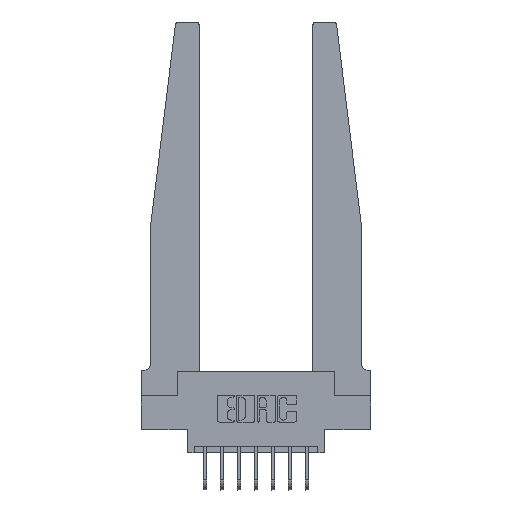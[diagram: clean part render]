
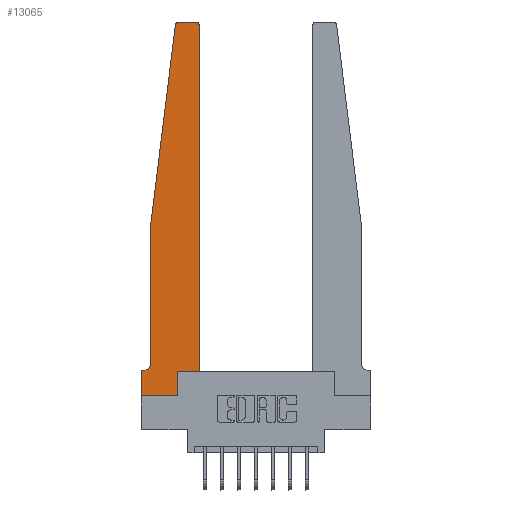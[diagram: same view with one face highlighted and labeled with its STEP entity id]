
A CAD part, top view. The second image highlights one B-rep face of the part: STEP entity #13065.
In plain terms, the highlighted planar face has unit normal (0, 0, 1).
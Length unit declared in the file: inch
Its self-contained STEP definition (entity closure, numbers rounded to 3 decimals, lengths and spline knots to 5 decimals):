
#137 = CARTESIAN_POINT ( 'NONE',  ( 0.425, 0.18, 0.37 ) ) ;
#297 = VERTEX_POINT ( 'NONE', #11031 ) ;
#320 = CIRCLE ( 'NONE', #13896, 0.05 ) ;
#441 = CIRCLE ( 'NONE', #13308, 0.03 ) ;
#601 = CARTESIAN_POINT ( 'NONE',  ( 0.2605, 0., 0.37 ) ) ;
#698 = EDGE_CURVE ( 'NONE', #11782, #7622, #10846, .T. ) ;
#818 = LINE ( 'NONE', #1901, #2345 ) ;
#869 = DIRECTION ( 'NONE',  ( -1., 0., 0. ) ) ;
#914 = CARTESIAN_POINT ( 'NONE',  ( 0.015, 0.1875, 0.37 ) ) ;
#1117 = EDGE_LOOP ( 'NONE', ( #6848, #2560, #4452, #10578, #6631, #8452, #12022, #9061, #5543, #2909, #1561, #4451 ) ) ;
#1201 = DIRECTION ( 'NONE',  ( 0., 1., 0. ) ) ;
#1331 = DIRECTION ( 'NONE',  ( 0., 0., 1. ) ) ;
#1561 = ORIENTED_EDGE ( 'NONE', *, *, #6598, .T. ) ;
#1574 = DIRECTION ( 'NONE',  ( 0., 0., 1. ) ) ;
#1683 = EDGE_CURVE ( 'NONE', #4079, #10030, #320, .T. ) ;
#1731 = VECTOR ( 'NONE', #9691, 39.37008 ) ;
#1901 = CARTESIAN_POINT ( 'NONE',  ( 0.425, 0.18, 0.37 ) ) ;
#2051 = CARTESIAN_POINT ( 'NONE',  ( 0.25, 2.75, 0.37 ) ) ;
#2220 = CARTESIAN_POINT ( 'NONE',  ( 0.395, 2.75, 0.37 ) ) ;
#2345 = VECTOR ( 'NONE', #6035, 39.37008 ) ;
#2426 = PLANE ( 'NONE',  #11537 ) ;
#2560 = ORIENTED_EDGE ( 'NONE', *, *, #6254, .T. ) ;
#2582 = CARTESIAN_POINT ( 'NONE',  ( 0., 0., 0.37 ) ) ;
#2596 = VECTOR ( 'NONE', #9043, 39.37008 ) ;
#2607 = VECTOR ( 'NONE', #13675, 39.37008 ) ;
#2705 = DIRECTION ( 'NONE',  ( 1., 0., 0. ) ) ;
#2909 = ORIENTED_EDGE ( 'NONE', *, *, #5904, .T. ) ;
#3220 = CARTESIAN_POINT ( 'NONE',  ( 0.065, 0.1875, 0.37 ) ) ;
#3271 = CARTESIAN_POINT ( 'NONE',  ( 0.015, 0.2375, 0.37 ) ) ;
#3797 = CARTESIAN_POINT ( 'NONE',  ( 0.27653, 2.72, 0.37 ) ) ;
#3983 = EDGE_CURVE ( 'NONE', #10411, #13449, #12969, .T. ) ;
#4079 = VERTEX_POINT ( 'NONE', #7240 ) ;
#4344 = EDGE_CURVE ( 'NONE', #10246, #8639, #9429, .T. ) ;
#4451 = ORIENTED_EDGE ( 'NONE', *, *, #698, .T. ) ;
#4452 = ORIENTED_EDGE ( 'NONE', *, *, #3983, .T. ) ;
#4714 = LINE ( 'NONE', #5595, #13390 ) ;
#4793 = DIRECTION ( 'NONE',  ( 0., -1., 0. ) ) ;
#5105 = DIRECTION ( 'NONE',  ( -0.122, -0.992, 0. ) ) ;
#5543 = ORIENTED_EDGE ( 'NONE', *, *, #10256, .T. ) ;
#5595 = CARTESIAN_POINT ( 'NONE',  ( 0.2605, 0.18, 0.37 ) ) ;
#5759 = CARTESIAN_POINT ( 'NONE',  ( 0., 0., 0.37 ) ) ;
#5762 = CARTESIAN_POINT ( 'NONE',  ( 0., 0., 0.37 ) ) ;
#5813 = CARTESIAN_POINT ( 'NONE',  ( 0., 0.1875, 0.37 ) ) ;
#5904 = EDGE_CURVE ( 'NONE', #14384, #6146, #818, .T. ) ;
#6035 = DIRECTION ( 'NONE',  ( 1., 0., 0. ) ) ;
#6146 = VERTEX_POINT ( 'NONE', #12535 ) ;
#6254 = EDGE_CURVE ( 'NONE', #297, #10411, #441, .T. ) ;
#6594 = LINE ( 'NONE', #2051, #1731 ) ;
#6598 = EDGE_CURVE ( 'NONE', #6146, #11782, #11642, .T. ) ;
#6631 = ORIENTED_EDGE ( 'NONE', *, *, #1683, .T. ) ;
#6680 = LINE ( 'NONE', #3220, #2596 ) ;
#6848 = ORIENTED_EDGE ( 'NONE', *, *, #14464, .T. ) ;
#6965 = DIRECTION ( 'NONE',  ( 1., 0., 0. ) ) ;
#7240 = CARTESIAN_POINT ( 'NONE',  ( 0.065, 0.2375, 0.37 ) ) ;
#7296 = EDGE_CURVE ( 'NONE', #13449, #4079, #12188, .T. ) ;
#7355 = CARTESIAN_POINT ( 'NONE',  ( 0.24675, 2.72367, 0.37 ) ) ;
#7622 = VERTEX_POINT ( 'NONE', #2220 ) ;
#7782 = VERTEX_POINT ( 'NONE', #601 ) ;
#7886 = LINE ( 'NONE', #5762, #2607 ) ;
#8452 = ORIENTED_EDGE ( 'NONE', *, *, #9415, .T. ) ;
#8639 = VERTEX_POINT ( 'NONE', #5759 ) ;
#9043 = DIRECTION ( 'NONE',  ( -1., 0., 0. ) ) ;
#9061 = ORIENTED_EDGE ( 'NONE', *, *, #9825, .T. ) ;
#9120 = CARTESIAN_POINT ( 'NONE',  ( 0., 0.1875, 0.37 ) ) ;
#9155 = DIRECTION ( 'NONE',  ( 0., 1., 0. ) ) ;
#9415 = EDGE_CURVE ( 'NONE', #10030, #10246, #6680, .T. ) ;
#9429 = LINE ( 'NONE', #2582, #12612 ) ;
#9691 = DIRECTION ( 'NONE',  ( -1., 0., 0. ) ) ;
#9775 = DIRECTION ( 'NONE',  ( 0., -1., 0. ) ) ;
#9825 = EDGE_CURVE ( 'NONE', #8639, #7782, #7886, .T. ) ;
#10030 = VERTEX_POINT ( 'NONE', #914 ) ;
#10033 = VECTOR ( 'NONE', #9155, 39.37008 ) ;
#10246 = VERTEX_POINT ( 'NONE', #5813 ) ;
#10256 = EDGE_CURVE ( 'NONE', #7782, #14384, #4714, .T. ) ;
#10411 = VERTEX_POINT ( 'NONE', #7355 ) ;
#10578 = ORIENTED_EDGE ( 'NONE', *, *, #7296, .T. ) ;
#10663 = CARTESIAN_POINT ( 'NONE',  ( 0.2605, 0.18, 0.37 ) ) ;
#10846 = CIRCLE ( 'NONE', #11767, 0.03 ) ;
#11031 = CARTESIAN_POINT ( 'NONE',  ( 0.27653, 2.75, 0.37 ) ) ;
#11180 = CARTESIAN_POINT ( 'NONE',  ( 0.065, 1.25, 0.37 ) ) ;
#11315 = CARTESIAN_POINT ( 'NONE',  ( 0.425, 2.72, 0.37 ) ) ;
#11385 = FACE_OUTER_BOUND ( 'NONE', #1117, .T. ) ;
#11537 = AXIS2_PLACEMENT_3D ( 'NONE', #9120, #1331, #6965 ) ;
#11642 = LINE ( 'NONE', #137, #10033 ) ;
#11654 = CARTESIAN_POINT ( 'NONE',  ( 0.065, 1.25, 0.37 ) ) ;
#11696 = DIRECTION ( 'NONE',  ( 1., 0., 0. ) ) ;
#11767 = AXIS2_PLACEMENT_3D ( 'NONE', #12505, #1574, #11696 ) ;
#11782 = VERTEX_POINT ( 'NONE', #11315 ) ;
#12022 = ORIENTED_EDGE ( 'NONE', *, *, #4344, .T. ) ;
#12188 = LINE ( 'NONE', #11180, #12863 ) ;
#12505 = CARTESIAN_POINT ( 'NONE',  ( 0.395, 2.72, 0.37 ) ) ;
#12535 = CARTESIAN_POINT ( 'NONE',  ( 0.425, 0.18, 0.37 ) ) ;
#12612 = VECTOR ( 'NONE', #4793, 39.37008 ) ;
#12740 = VECTOR ( 'NONE', #5105, 39.37008 ) ;
#12749 = DIRECTION ( 'NONE',  ( 0., 0., 1. ) ) ;
#12863 = VECTOR ( 'NONE', #9775, 39.37008 ) ;
#12969 = LINE ( 'NONE', #11654, #12740 ) ;
#13065 = ADVANCED_FACE ( 'NONE', ( #11385 ), #2426, .T. ) ;
#13260 = DIRECTION ( 'NONE',  ( 0., 0., -1. ) ) ;
#13308 = AXIS2_PLACEMENT_3D ( 'NONE', #3797, #12749, #2705 ) ;
#13390 = VECTOR ( 'NONE', #1201, 39.37008 ) ;
#13449 = VERTEX_POINT ( 'NONE', #13547 ) ;
#13547 = CARTESIAN_POINT ( 'NONE',  ( 0.065, 1.25, 0.37 ) ) ;
#13675 = DIRECTION ( 'NONE',  ( 1., 0., 0. ) ) ;
#13896 = AXIS2_PLACEMENT_3D ( 'NONE', #3271, #13260, #869 ) ;
#14384 = VERTEX_POINT ( 'NONE', #10663 ) ;
#14464 = EDGE_CURVE ( 'NONE', #7622, #297, #6594, .T. ) ;
